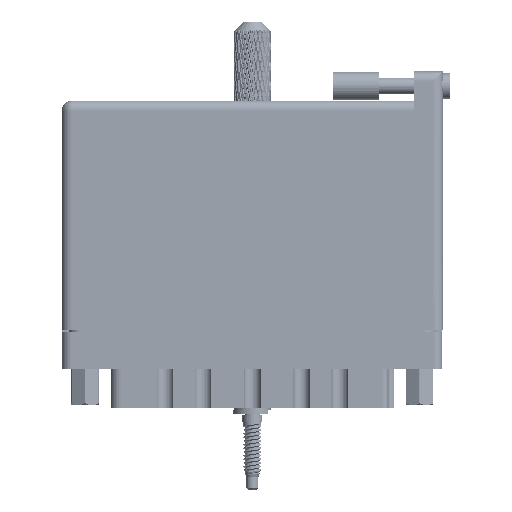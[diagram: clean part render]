
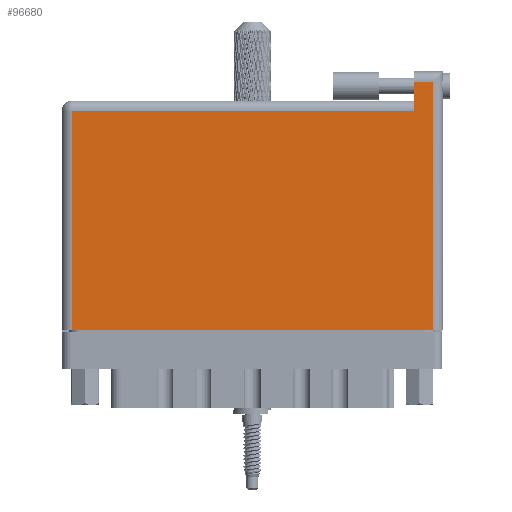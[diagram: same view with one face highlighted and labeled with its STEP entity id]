
A CAD part, front view. The second image highlights one B-rep face of the part: STEP entity #96680.
In plain terms, the highlighted face is planar.
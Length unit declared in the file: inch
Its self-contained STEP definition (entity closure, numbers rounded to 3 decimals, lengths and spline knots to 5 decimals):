
#4295 = CARTESIAN_POINT ( 'NONE',  ( 0., 1.566, 0. ) ) ;
#4714 = CARTESIAN_POINT ( 'NONE',  ( 2.53, 1.696, 0. ) ) ;
#6011 = CARTESIAN_POINT ( 'NONE',  ( 2.403, 1.766, 0. ) ) ;
#10682 = FACE_OUTER_BOUND ( 'NONE', #101062, .T. ) ;
#13337 = LINE ( 'NONE', #99085, #65764 ) ;
#14729 = EDGE_CURVE ( 'NONE', #70438, #89653, #13337, .T. ) ;
#19017 = VECTOR ( 'NONE', #48790, 39.37008 ) ;
#22560 = EDGE_CURVE ( 'NONE', #50875, #90654, #121573, .T. ) ;
#23052 = CARTESIAN_POINT ( 'NONE',  ( 2.403, 1.496, 0. ) ) ;
#29567 = DIRECTION ( 'NONE',  ( 0., -1., 0. ) ) ;
#30208 = CARTESIAN_POINT ( 'NONE',  ( 0.07, 0., 0. ) ) ;
#30380 = VERTEX_POINT ( 'NONE', #39847 ) ;
#33678 = ORIENTED_EDGE ( 'NONE', *, *, #78430, .T. ) ;
#36406 = CARTESIAN_POINT ( 'NONE',  ( 0., 0., 0. ) ) ;
#37870 = ORIENTED_EDGE ( 'NONE', *, *, #117066, .T. ) ;
#39847 = CARTESIAN_POINT ( 'NONE',  ( 0.07, 0., 0. ) ) ;
#40005 = DIRECTION ( 'NONE',  ( -1., 0., 0. ) ) ;
#40754 = DIRECTION ( 'NONE',  ( 1., 0., 0. ) ) ;
#43156 = LINE ( 'NONE', #6011, #104837 ) ;
#44512 = LINE ( 'NONE', #36406, #126253 ) ;
#46305 = ORIENTED_EDGE ( 'NONE', *, *, #127499, .T. ) ;
#47882 = VECTOR ( 'NONE', #121761, 39.37008 ) ;
#48790 = DIRECTION ( 'NONE',  ( 0., -1., 0. ) ) ;
#50093 = ORIENTED_EDGE ( 'NONE', *, *, #22560, .T. ) ;
#50875 = VERTEX_POINT ( 'NONE', #4714 ) ;
#53601 = ORIENTED_EDGE ( 'NONE', *, *, #14729, .T. ) ;
#63381 = PLANE ( 'NONE',  #86896 ) ;
#64644 = DIRECTION ( 'NONE',  ( -1., 0., 0. ) ) ;
#65764 = VECTOR ( 'NONE', #40005, 39.37008 ) ;
#68586 = VERTEX_POINT ( 'NONE', #86085 ) ;
#70438 = VERTEX_POINT ( 'NONE', #23052 ) ;
#78430 = EDGE_CURVE ( 'NONE', #68586, #50875, #86474, .T. ) ;
#86085 = CARTESIAN_POINT ( 'NONE',  ( 2.53, 0., 0. ) ) ;
#86474 = LINE ( 'NONE', #99037, #47882 ) ;
#86896 = AXIS2_PLACEMENT_3D ( 'NONE', #4295, #114182, #64644 ) ;
#87132 = ORIENTED_EDGE ( 'NONE', *, *, #115137, .T. ) ;
#89653 = VERTEX_POINT ( 'NONE', #116941 ) ;
#90654 = VERTEX_POINT ( 'NONE', #96607 ) ;
#93818 = DIRECTION ( 'NONE',  ( -1., 0., 0. ) ) ;
#96607 = CARTESIAN_POINT ( 'NONE',  ( 2.403, 1.696, 0. ) ) ;
#96680 = ADVANCED_FACE ( 'NONE', ( #10682 ), #63381, .F. ) ;
#99037 = CARTESIAN_POINT ( 'NONE',  ( 2.53, 1.766, 0. ) ) ;
#99085 = CARTESIAN_POINT ( 'NONE',  ( 0., 1.496, 0. ) ) ;
#101062 = EDGE_LOOP ( 'NONE', ( #37870, #33678, #50093, #87132, #53601, #46305 ) ) ;
#101632 = CARTESIAN_POINT ( 'NONE',  ( 0., 1.696, 0. ) ) ;
#104837 = VECTOR ( 'NONE', #29567, 39.37008 ) ;
#109217 = VECTOR ( 'NONE', #93818, 39.37008 ) ;
#109949 = LINE ( 'NONE', #30208, #19017 ) ;
#114182 = DIRECTION ( 'NONE',  ( 0., 0., -1. ) ) ;
#115137 = EDGE_CURVE ( 'NONE', #90654, #70438, #43156, .T. ) ;
#116941 = CARTESIAN_POINT ( 'NONE',  ( 0.07, 1.496, 0. ) ) ;
#117066 = EDGE_CURVE ( 'NONE', #30380, #68586, #44512, .T. ) ;
#121573 = LINE ( 'NONE', #101632, #109217 ) ;
#121761 = DIRECTION ( 'NONE',  ( 0., 1., 0. ) ) ;
#126253 = VECTOR ( 'NONE', #40754, 39.37008 ) ;
#127499 = EDGE_CURVE ( 'NONE', #89653, #30380, #109949, .T. ) ;
